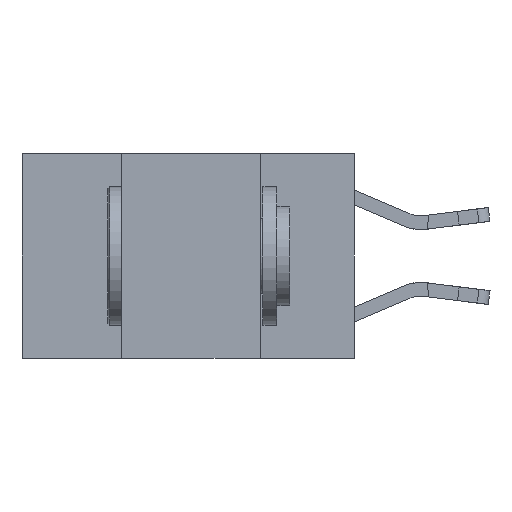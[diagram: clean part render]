
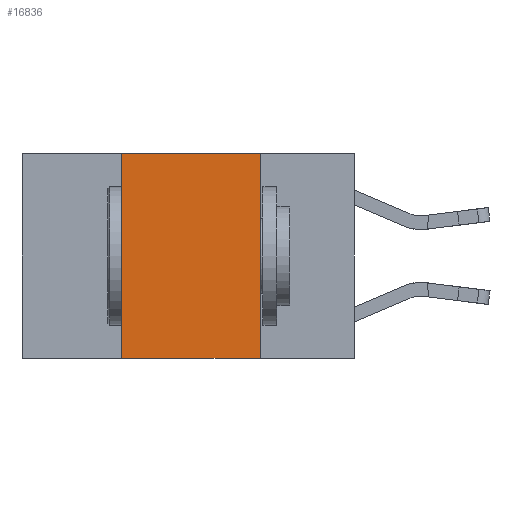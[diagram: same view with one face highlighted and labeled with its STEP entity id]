
A CAD part, left-side view. The second image highlights one B-rep face of the part: STEP entity #16836.
In plain terms, the highlighted planar face has unit normal (-1, 0, 0).
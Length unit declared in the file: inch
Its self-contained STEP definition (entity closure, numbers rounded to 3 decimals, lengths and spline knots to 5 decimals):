
#59 = VERTEX_POINT ( 'NONE', #8842 ) ;
#561 = ORIENTED_EDGE ( 'NONE', *, *, #7228, .F. ) ;
#1046 = ORIENTED_EDGE ( 'NONE', *, *, #13416, .F. ) ;
#2873 = PLANE ( 'NONE',  #13785 ) ;
#4363 = CARTESIAN_POINT ( 'NONE',  ( 0., 0.17, -0.37 ) ) ;
#4448 = CARTESIAN_POINT ( 'NONE',  ( 0., 0.6, 0. ) ) ;
#5097 = VERTEX_POINT ( 'NONE', #4363 ) ;
#5336 = LINE ( 'NONE', #11731, #19984 ) ;
#5678 = CARTESIAN_POINT ( 'NONE',  ( 0., 0.6, 0. ) ) ;
#5780 = DIRECTION ( 'NONE',  ( 0., -1., 0. ) ) ;
#6154 = DIRECTION ( 'NONE',  ( 0., 0., 1. ) ) ;
#7092 = VECTOR ( 'NONE', #13169, 39.37008 ) ;
#7115 = VECTOR ( 'NONE', #5780, 39.37008 ) ;
#7228 = EDGE_CURVE ( 'NONE', #10481, #8734, #14110, .T. ) ;
#8306 = CARTESIAN_POINT ( 'NONE',  ( 0., 0.42, -0.37 ) ) ;
#8734 = VERTEX_POINT ( 'NONE', #18098 ) ;
#8842 = CARTESIAN_POINT ( 'NONE',  ( 0., 0.17, 0. ) ) ;
#9290 = EDGE_CURVE ( 'NONE', #10481, #5097, #5336, .T. ) ;
#10142 = ORIENTED_EDGE ( 'NONE', *, *, #9290, .T. ) ;
#10481 = VERTEX_POINT ( 'NONE', #8306 ) ;
#11731 = CARTESIAN_POINT ( 'NONE',  ( 0., 0.6, -0.37 ) ) ;
#11971 = EDGE_LOOP ( 'NONE', ( #1046, #15910, #561, #10142 ) ) ;
#12953 = LINE ( 'NONE', #17952, #7092 ) ;
#13169 = DIRECTION ( 'NONE',  ( 0., 0., -1. ) ) ;
#13416 = EDGE_CURVE ( 'NONE', #59, #5097, #12953, .T. ) ;
#13785 = AXIS2_PLACEMENT_3D ( 'NONE', #4448, #20062, #15447 ) ;
#14110 = LINE ( 'NONE', #20461, #20277 ) ;
#15079 = LINE ( 'NONE', #5678, #7115 ) ;
#15447 = DIRECTION ( 'NONE',  ( 0., 0., -1. ) ) ;
#15910 = ORIENTED_EDGE ( 'NONE', *, *, #15993, .F. ) ;
#15993 = EDGE_CURVE ( 'NONE', #8734, #59, #15079, .T. ) ;
#16836 = ADVANCED_FACE ( 'NONE', ( #19965 ), #2873, .F. ) ;
#17952 = CARTESIAN_POINT ( 'NONE',  ( 0., 0.17, 0. ) ) ;
#18072 = DIRECTION ( 'NONE',  ( 0., -1., 0. ) ) ;
#18098 = CARTESIAN_POINT ( 'NONE',  ( 0., 0.42, 0. ) ) ;
#19965 = FACE_OUTER_BOUND ( 'NONE', #11971, .T. ) ;
#19984 = VECTOR ( 'NONE', #18072, 39.37008 ) ;
#20062 = DIRECTION ( 'NONE',  ( 1., 0., 0. ) ) ;
#20277 = VECTOR ( 'NONE', #6154, 39.37008 ) ;
#20461 = CARTESIAN_POINT ( 'NONE',  ( 0., 0.42, 0. ) ) ;
